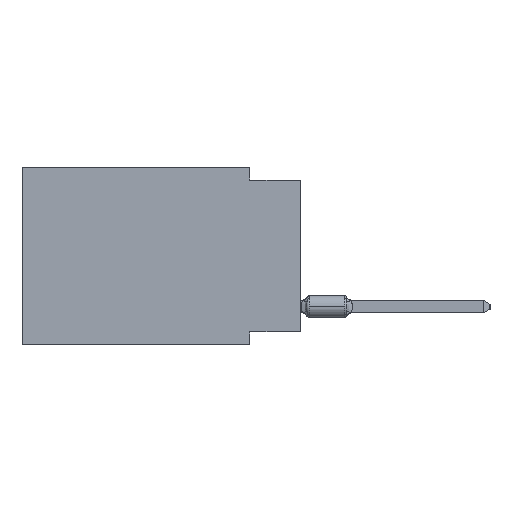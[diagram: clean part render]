
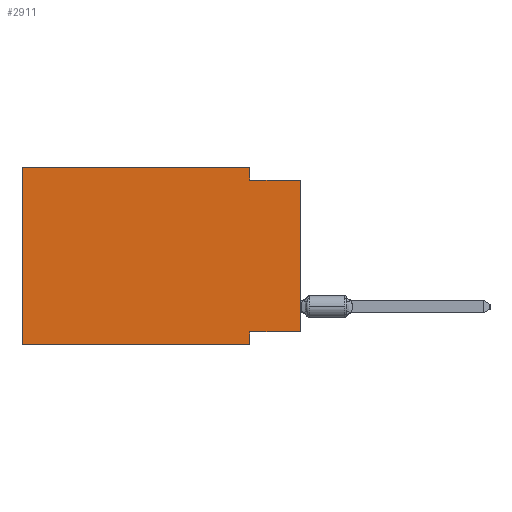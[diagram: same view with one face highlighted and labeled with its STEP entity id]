
A CAD part, left-side view. The second image highlights one B-rep face of the part: STEP entity #2911.
In plain terms, the highlighted planar face has unit normal (-1, 0, 0).
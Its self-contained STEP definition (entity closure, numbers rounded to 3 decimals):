
#1269 = CARTESIAN_POINT ( 'NONE',  ( 0., 0., -8.255 ) ) ;
#1516 = VECTOR ( 'NONE', #24899, 1000. ) ;
#2911 = ADVANCED_FACE ( 'NONE', ( #16165 ), #26747, .F. ) ;
#4525 = CARTESIAN_POINT ( 'NONE',  ( 0., 13.97, 0. ) ) ;
#6363 = CARTESIAN_POINT ( 'NONE',  ( 0., 13.97, 0. ) ) ;
#7117 = CARTESIAN_POINT ( 'NONE',  ( 0., 0., -0.635 ) ) ;
#9347 = DIRECTION ( 'NONE',  ( 0., 0., -1. ) ) ;
#9792 = EDGE_CURVE ( 'NONE', #12024, #51222, #35139, .T. ) ;
#10292 = DIRECTION ( 'NONE',  ( 0., 0., -1. ) ) ;
#10660 = DIRECTION ( 'NONE',  ( 1., 0., 0. ) ) ;
#11362 = ORIENTED_EDGE ( 'NONE', *, *, #59186, .F. ) ;
#12024 = VERTEX_POINT ( 'NONE', #55578 ) ;
#12453 = ORIENTED_EDGE ( 'NONE', *, *, #37149, .F. ) ;
#12491 = DIRECTION ( 'NONE',  ( 0., -1., 0. ) ) ;
#12842 = EDGE_CURVE ( 'NONE', #54291, #48277, #49930, .T. ) ;
#14175 = CARTESIAN_POINT ( 'NONE',  ( 0., 2.54, -8.89 ) ) ;
#14458 = ORIENTED_EDGE ( 'NONE', *, *, #9792, .T. ) ;
#15597 = DIRECTION ( 'NONE',  ( 0., 0., 1. ) ) ;
#16165 = FACE_OUTER_BOUND ( 'NONE', #26347, .T. ) ;
#17128 = ORIENTED_EDGE ( 'NONE', *, *, #34774, .F. ) ;
#18134 = VECTOR ( 'NONE', #54402, 1000. ) ;
#18158 = VECTOR ( 'NONE', #9347, 1000. ) ;
#19720 = LINE ( 'NONE', #62397, #53575 ) ;
#19924 = DIRECTION ( 'NONE',  ( 0., 0., -1. ) ) ;
#20809 = CARTESIAN_POINT ( 'NONE',  ( 0., 13.97, -8.89 ) ) ;
#20983 = VECTOR ( 'NONE', #22135, 1000. ) ;
#22135 = DIRECTION ( 'NONE',  ( 0., 1., 0. ) ) ;
#24899 = DIRECTION ( 'NONE',  ( 0., 0., 1. ) ) ;
#25000 = ORIENTED_EDGE ( 'NONE', *, *, #27903, .F. ) ;
#25403 = ORIENTED_EDGE ( 'NONE', *, *, #35746, .F. ) ;
#26347 = EDGE_LOOP ( 'NONE', ( #14458, #25000, #17128, #25403, #12453, #30212, #48579, #11362 ) ) ;
#26747 = PLANE ( 'NONE',  #48864 ) ;
#27903 = EDGE_CURVE ( 'NONE', #42395, #51222, #38575, .T. ) ;
#30212 = ORIENTED_EDGE ( 'NONE', *, *, #12842, .T. ) ;
#31051 = VECTOR ( 'NONE', #54281, 1000. ) ;
#32063 = CARTESIAN_POINT ( 'NONE',  ( 0., 13.97, 0. ) ) ;
#34774 = EDGE_CURVE ( 'NONE', #35661, #42395, #52004, .T. ) ;
#35139 = LINE ( 'NONE', #45066, #1516 ) ;
#35661 = VERTEX_POINT ( 'NONE', #40899 ) ;
#35746 = EDGE_CURVE ( 'NONE', #40509, #35661, #37465, .T. ) ;
#37149 = EDGE_CURVE ( 'NONE', #54291, #40509, #19720, .T. ) ;
#37312 = CARTESIAN_POINT ( 'NONE',  ( 0., 2.54, 0. ) ) ;
#37465 = LINE ( 'NONE', #6363, #43374 ) ;
#38575 = LINE ( 'NONE', #7117, #31051 ) ;
#38876 = VECTOR ( 'NONE', #10292, 1000. ) ;
#39029 = CARTESIAN_POINT ( 'NONE',  ( 0., 13.97, -8.89 ) ) ;
#39969 = CARTESIAN_POINT ( 'NONE',  ( 0., 2.54, -0.635 ) ) ;
#40509 = VERTEX_POINT ( 'NONE', #32063 ) ;
#40899 = CARTESIAN_POINT ( 'NONE',  ( 0., 2.54, 0. ) ) ;
#42395 = VERTEX_POINT ( 'NONE', #39969 ) ;
#43374 = VECTOR ( 'NONE', #12491, 1000. ) ;
#45066 = CARTESIAN_POINT ( 'NONE',  ( 0., 0., 0. ) ) ;
#48277 = VERTEX_POINT ( 'NONE', #58355 ) ;
#48579 = ORIENTED_EDGE ( 'NONE', *, *, #64042, .F. ) ;
#48864 = AXIS2_PLACEMENT_3D ( 'NONE', #4525, #10660, #19924 ) ;
#49930 = LINE ( 'NONE', #39029, #18134 ) ;
#50627 = VERTEX_POINT ( 'NONE', #56495 ) ;
#51222 = VERTEX_POINT ( 'NONE', #60122 ) ;
#52004 = LINE ( 'NONE', #37312, #38876 ) ;
#53575 = VECTOR ( 'NONE', #15597, 1000. ) ;
#54281 = DIRECTION ( 'NONE',  ( 0., -1., 0. ) ) ;
#54291 = VERTEX_POINT ( 'NONE', #20809 ) ;
#54402 = DIRECTION ( 'NONE',  ( 0., -1., 0. ) ) ;
#55578 = CARTESIAN_POINT ( 'NONE',  ( 0., 0., -8.255 ) ) ;
#56495 = CARTESIAN_POINT ( 'NONE',  ( 0., 2.54, -8.255 ) ) ;
#58355 = CARTESIAN_POINT ( 'NONE',  ( 0., 2.54, -8.89 ) ) ;
#58358 = LINE ( 'NONE', #1269, #20983 ) ;
#59186 = EDGE_CURVE ( 'NONE', #12024, #50627, #58358, .T. ) ;
#60122 = CARTESIAN_POINT ( 'NONE',  ( 0., 0., -0.635 ) ) ;
#62397 = CARTESIAN_POINT ( 'NONE',  ( 0., 13.97, 0. ) ) ;
#64042 = EDGE_CURVE ( 'NONE', #50627, #48277, #67082, .T. ) ;
#67082 = LINE ( 'NONE', #14175, #18158 ) ;
